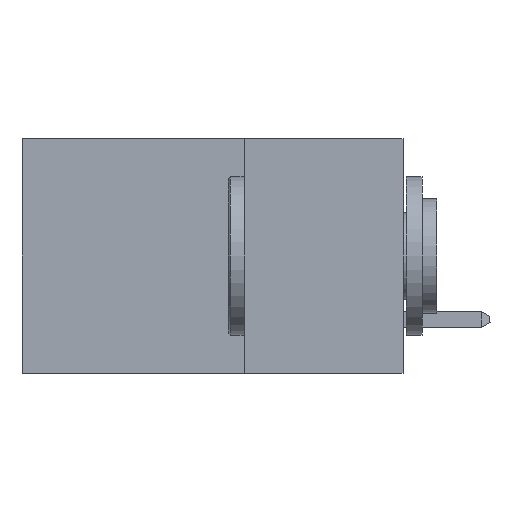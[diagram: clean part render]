
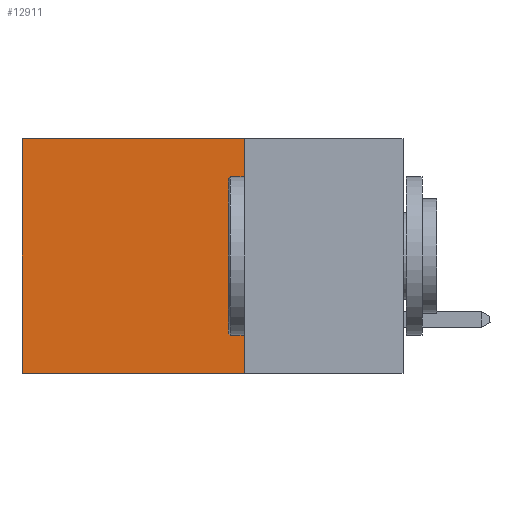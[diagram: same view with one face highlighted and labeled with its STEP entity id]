
A CAD part, left-side view. The second image highlights one B-rep face of the part: STEP entity #12911.
In plain terms, the highlighted planar face has unit normal (-1, 0, 0).
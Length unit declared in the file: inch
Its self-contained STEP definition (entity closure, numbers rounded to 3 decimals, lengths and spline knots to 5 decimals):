
#1712 = CARTESIAN_POINT ( 'NONE',  ( 0.2875, 0.25, 0. ) ) ;
#1903 = DIRECTION ( 'NONE',  ( 0., 0., -1. ) ) ;
#3077 = CARTESIAN_POINT ( 'NONE',  ( 0.2875, 0.6, 0. ) ) ;
#3941 = VERTEX_POINT ( 'NONE', #7508 ) ;
#4358 = ORIENTED_EDGE ( 'NONE', *, *, #6616, .F. ) ;
#4573 = DIRECTION ( 'NONE',  ( 0., 1., 0. ) ) ;
#4983 = VECTOR ( 'NONE', #9948, 39.37008 ) ;
#5803 = CARTESIAN_POINT ( 'NONE',  ( 0.2875, 0.25, -0.37 ) ) ;
#6056 = EDGE_LOOP ( 'NONE', ( #13058, #9533, #4358, #8189 ) ) ;
#6616 = EDGE_CURVE ( 'NONE', #15834, #7607, #15789, .T. ) ;
#7253 = CARTESIAN_POINT ( 'NONE',  ( 0.2875, 0.25, 0. ) ) ;
#7508 = CARTESIAN_POINT ( 'NONE',  ( 0.2875, 0.6, 0. ) ) ;
#7607 = VERTEX_POINT ( 'NONE', #5803 ) ;
#8189 = ORIENTED_EDGE ( 'NONE', *, *, #15598, .T. ) ;
#8499 = LINE ( 'NONE', #16059, #11702 ) ;
#9476 = VECTOR ( 'NONE', #4573, 39.37008 ) ;
#9533 = ORIENTED_EDGE ( 'NONE', *, *, #10654, .F. ) ;
#9948 = DIRECTION ( 'NONE',  ( 0., 0., -1. ) ) ;
#9989 = DIRECTION ( 'NONE',  ( 1., 0., 0. ) ) ;
#10163 = PLANE ( 'NONE',  #14176 ) ;
#10654 = EDGE_CURVE ( 'NONE', #7607, #10771, #16677, .T. ) ;
#10771 = VERTEX_POINT ( 'NONE', #12980 ) ;
#11508 = EDGE_CURVE ( 'NONE', #3941, #10771, #16834, .T. ) ;
#11702 = VECTOR ( 'NONE', #14754, 39.37008 ) ;
#12911 = ADVANCED_FACE ( 'NONE', ( #14675 ), #10163, .F. ) ;
#12919 = CARTESIAN_POINT ( 'NONE',  ( 0.2875, 0.25, -0.37 ) ) ;
#12980 = CARTESIAN_POINT ( 'NONE',  ( 0.2875, 0.6, -0.37 ) ) ;
#13058 = ORIENTED_EDGE ( 'NONE', *, *, #11508, .T. ) ;
#13940 = CARTESIAN_POINT ( 'NONE',  ( 0.2875, 0.25, 0. ) ) ;
#14176 = AXIS2_PLACEMENT_3D ( 'NONE', #7253, #9989, #1903 ) ;
#14675 = FACE_OUTER_BOUND ( 'NONE', #6056, .T. ) ;
#14754 = DIRECTION ( 'NONE',  ( 0., 1., 0. ) ) ;
#15144 = VECTOR ( 'NONE', #16868, 39.37008 ) ;
#15598 = EDGE_CURVE ( 'NONE', #15834, #3941, #8499, .T. ) ;
#15789 = LINE ( 'NONE', #13940, #15144 ) ;
#15834 = VERTEX_POINT ( 'NONE', #1712 ) ;
#16059 = CARTESIAN_POINT ( 'NONE',  ( 0.2875, 0.25, 0. ) ) ;
#16677 = LINE ( 'NONE', #12919, #9476 ) ;
#16834 = LINE ( 'NONE', #3077, #4983 ) ;
#16868 = DIRECTION ( 'NONE',  ( 0., 0., -1. ) ) ;
